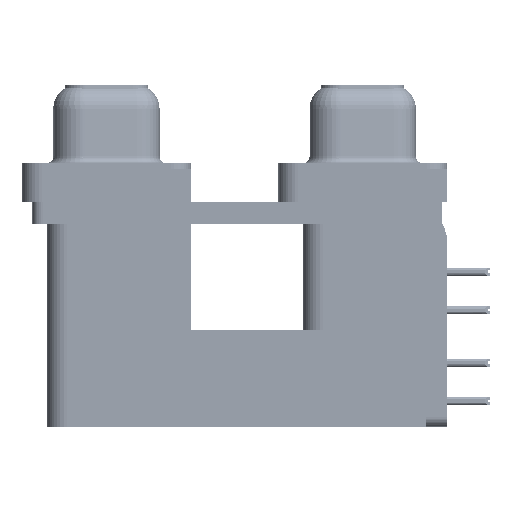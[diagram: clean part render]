
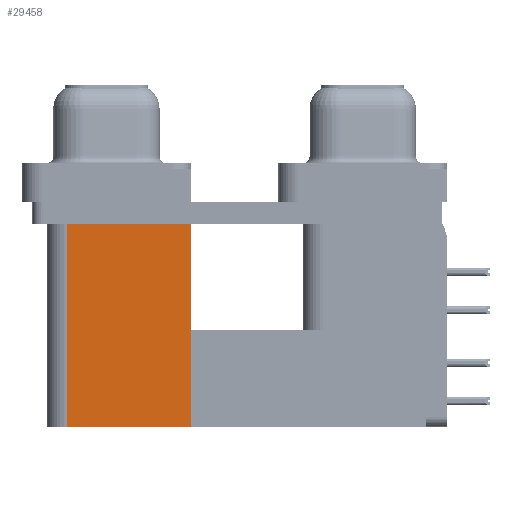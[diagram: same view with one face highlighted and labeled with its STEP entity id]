
A CAD part, left-side view. The second image highlights one B-rep face of the part: STEP entity #29458.
In plain terms, the highlighted planar face has unit normal (-1, 0, 0).
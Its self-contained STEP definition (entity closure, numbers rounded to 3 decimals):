
#3708 = VECTOR ( 'NONE', #37650, 1000. ) ;
#5020 = CARTESIAN_POINT ( 'NONE',  ( 3.79, 21.975, -19.2 ) ) ;
#7268 = ORIENTED_EDGE ( 'NONE', *, *, #66755, .F. ) ;
#9444 = EDGE_LOOP ( 'NONE', ( #43006, #7268, #40294, #67154 ) ) ;
#9794 = VECTOR ( 'NONE', #40278, 1000. ) ;
#10435 = CARTESIAN_POINT ( 'NONE',  ( 3.79, 12.775, -2.5 ) ) ;
#15419 = EDGE_CURVE ( 'NONE', #46078, #53688, #37939, .T. ) ;
#16740 = FACE_OUTER_BOUND ( 'NONE', #9444, .T. ) ;
#17857 = DIRECTION ( 'NONE',  ( 1., 0., 0. ) ) ;
#18068 = AXIS2_PLACEMENT_3D ( 'NONE', #69028, #17857, #18241 ) ;
#18241 = DIRECTION ( 'NONE',  ( 0., 0., -1. ) ) ;
#19725 = VERTEX_POINT ( 'NONE', #5020 ) ;
#22987 = CARTESIAN_POINT ( 'NONE',  ( 3.79, 12.775, -19.2 ) ) ;
#25988 = VECTOR ( 'NONE', #33412, 1000. ) ;
#26634 = DIRECTION ( 'NONE',  ( 0., 0., 1. ) ) ;
#28645 = LINE ( 'NONE', #22987, #9794 ) ;
#29184 = PLANE ( 'NONE',  #18068 ) ;
#29458 = ADVANCED_FACE ( 'NONE', ( #16740 ), #29184, .F. ) ;
#33276 = CARTESIAN_POINT ( 'NONE',  ( 3.79, 21.975, -2.5 ) ) ;
#33412 = DIRECTION ( 'NONE',  ( 0., 1., 0. ) ) ;
#36877 = CARTESIAN_POINT ( 'NONE',  ( 3.79, 12.775, -2.5 ) ) ;
#37650 = DIRECTION ( 'NONE',  ( 0., 0., 1. ) ) ;
#37939 = LINE ( 'NONE', #10435, #25988 ) ;
#38015 = LINE ( 'NONE', #66978, #3708 ) ;
#40278 = DIRECTION ( 'NONE',  ( 0., 1., 0. ) ) ;
#40294 = ORIENTED_EDGE ( 'NONE', *, *, #51321, .F. ) ;
#43006 = ORIENTED_EDGE ( 'NONE', *, *, #15419, .T. ) ;
#43540 = LINE ( 'NONE', #66500, #53519 ) ;
#46078 = VERTEX_POINT ( 'NONE', #36877 ) ;
#47717 = CARTESIAN_POINT ( 'NONE',  ( 3.79, 12.775, -19.2 ) ) ;
#48878 = EDGE_CURVE ( 'NONE', #51840, #46078, #38015, .T. ) ;
#51321 = EDGE_CURVE ( 'NONE', #51840, #19725, #28645, .T. ) ;
#51840 = VERTEX_POINT ( 'NONE', #47717 ) ;
#53519 = VECTOR ( 'NONE', #26634, 1000. ) ;
#53688 = VERTEX_POINT ( 'NONE', #33276 ) ;
#66500 = CARTESIAN_POINT ( 'NONE',  ( 3.79, 21.975, -19.2 ) ) ;
#66755 = EDGE_CURVE ( 'NONE', #19725, #53688, #43540, .T. ) ;
#66978 = CARTESIAN_POINT ( 'NONE',  ( 3.79, 12.775, -19.2 ) ) ;
#67154 = ORIENTED_EDGE ( 'NONE', *, *, #48878, .T. ) ;
#69028 = CARTESIAN_POINT ( 'NONE',  ( 3.79, 12.775, -19.2 ) ) ;
